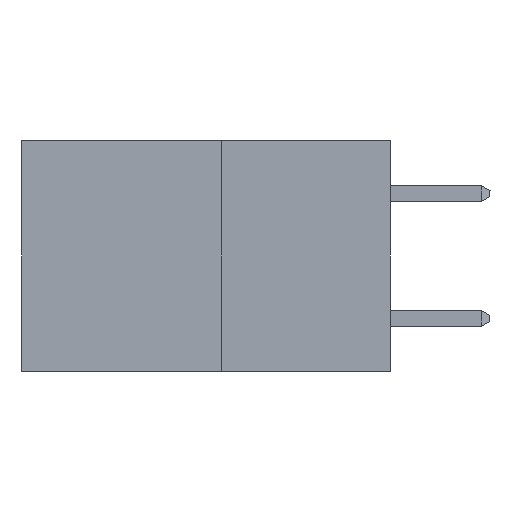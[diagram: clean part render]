
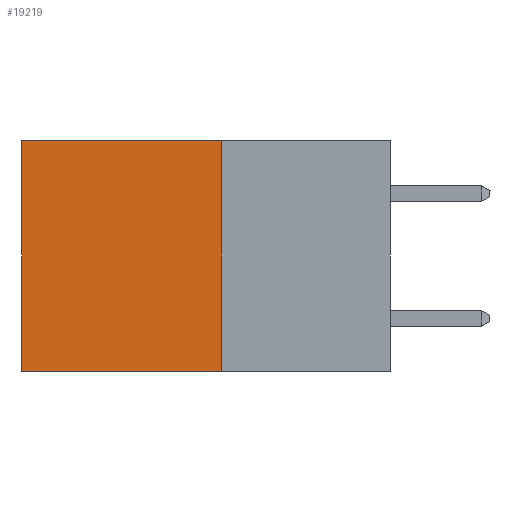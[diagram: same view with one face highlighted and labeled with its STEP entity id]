
A CAD part, left-side view. The second image highlights one B-rep face of the part: STEP entity #19219.
In plain terms, the highlighted planar face has unit normal (-1, 0, 0).
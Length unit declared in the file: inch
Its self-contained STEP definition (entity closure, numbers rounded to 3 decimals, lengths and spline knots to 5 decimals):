
#736 = EDGE_LOOP ( 'NONE', ( #5469, #15690, #5988, #1771 ) ) ;
#906 = EDGE_CURVE ( 'NONE', #8864, #17158, #6289, .T. ) ;
#1771 = ORIENTED_EDGE ( 'NONE', *, *, #906, .T. ) ;
#1840 = CARTESIAN_POINT ( 'NONE',  ( 0.277, 0.59, -0.37 ) ) ;
#4115 = CARTESIAN_POINT ( 'NONE',  ( 0.277, 0.59, 0. ) ) ;
#4522 = PLANE ( 'NONE',  #13496 ) ;
#5120 = LINE ( 'NONE', #19445, #8872 ) ;
#5469 = ORIENTED_EDGE ( 'NONE', *, *, #17490, .T. ) ;
#5988 = ORIENTED_EDGE ( 'NONE', *, *, #8435, .F. ) ;
#6289 = LINE ( 'NONE', #11483, #17387 ) ;
#6863 = LINE ( 'NONE', #11431, #18365 ) ;
#7099 = FACE_OUTER_BOUND ( 'NONE', #736, .T. ) ;
#8164 = LINE ( 'NONE', #1840, #16121 ) ;
#8435 = EDGE_CURVE ( 'NONE', #8864, #12063, #5120, .T. ) ;
#8453 = CARTESIAN_POINT ( 'NONE',  ( 0.277, 0.27, -0.37 ) ) ;
#8755 = CARTESIAN_POINT ( 'NONE',  ( 0.277, 0.59, -0.37 ) ) ;
#8864 = VERTEX_POINT ( 'NONE', #13898 ) ;
#8872 = VECTOR ( 'NONE', #19502, 39.37008 ) ;
#9034 = EDGE_CURVE ( 'NONE', #12063, #16383, #6863, .T. ) ;
#9329 = DIRECTION ( 'NONE',  ( 0., 0., -1. ) ) ;
#11431 = CARTESIAN_POINT ( 'NONE',  ( 0.277, 0.27, -0.37 ) ) ;
#11476 = DIRECTION ( 'NONE',  ( 0., 1., 0. ) ) ;
#11483 = CARTESIAN_POINT ( 'NONE',  ( 0.277, 0.27, 0. ) ) ;
#12063 = VERTEX_POINT ( 'NONE', #8453 ) ;
#12223 = CARTESIAN_POINT ( 'NONE',  ( 0.277, 0.27, -0.37 ) ) ;
#13496 = AXIS2_PLACEMENT_3D ( 'NONE', #12223, #18212, #9329 ) ;
#13898 = CARTESIAN_POINT ( 'NONE',  ( 0.277, 0.27, 0. ) ) ;
#15657 = DIRECTION ( 'NONE',  ( 0., 0., -1. ) ) ;
#15671 = DIRECTION ( 'NONE',  ( 0., 1., 0. ) ) ;
#15690 = ORIENTED_EDGE ( 'NONE', *, *, #9034, .F. ) ;
#16121 = VECTOR ( 'NONE', #15657, 39.37008 ) ;
#16383 = VERTEX_POINT ( 'NONE', #8755 ) ;
#17158 = VERTEX_POINT ( 'NONE', #4115 ) ;
#17387 = VECTOR ( 'NONE', #15671, 39.37008 ) ;
#17490 = EDGE_CURVE ( 'NONE', #17158, #16383, #8164, .T. ) ;
#18212 = DIRECTION ( 'NONE',  ( 1., 0., 0. ) ) ;
#18365 = VECTOR ( 'NONE', #11476, 39.37008 ) ;
#19219 = ADVANCED_FACE ( 'NONE', ( #7099 ), #4522, .F. ) ;
#19445 = CARTESIAN_POINT ( 'NONE',  ( 0.277, 0.27, -0.37 ) ) ;
#19502 = DIRECTION ( 'NONE',  ( 0., 0., -1. ) ) ;
